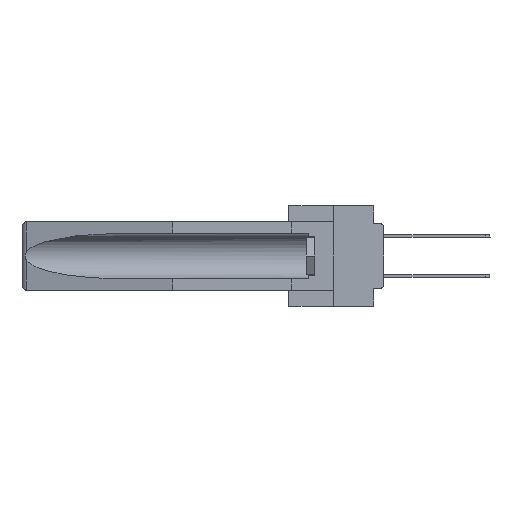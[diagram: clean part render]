
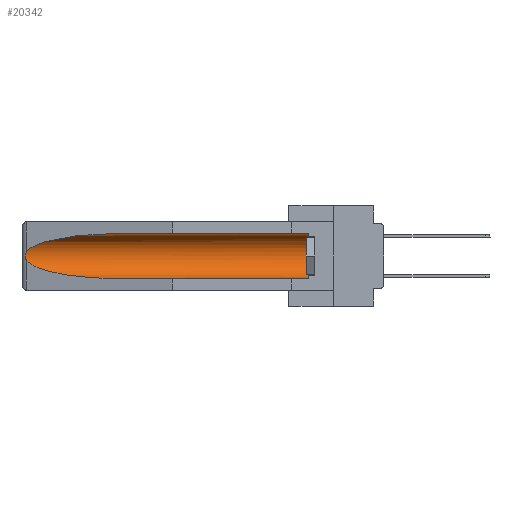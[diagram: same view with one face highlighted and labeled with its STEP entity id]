
A CAD part, left-side view. The second image highlights one B-rep face of the part: STEP entity #20342.
In plain terms, the highlighted cylindrical face has radius 2.857 mm (diameter 5.715 mm), a partial arc.
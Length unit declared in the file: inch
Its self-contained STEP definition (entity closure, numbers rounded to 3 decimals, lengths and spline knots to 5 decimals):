
#303 = CARTESIAN_POINT ( 'NONE',  ( 0.155, 1.07973, -0.284 ) ) ;
#502 = CARTESIAN_POINT ( 'NONE',  ( 0.26655, 1.53094, -0.18657 ) ) ;
#1109 = EDGE_CURVE ( 'NONE', #25879, #15699, #24027, .T. ) ;
#1837 = EDGE_CURVE ( 'NONE', #23606, #25879, #31931, .T. ) ;
#3815 = CARTESIAN_POINT ( 'NONE',  ( 0.2675, 1.53308, -0.17534 ) ) ;
#3900 = CARTESIAN_POINT ( 'NONE',  ( 0.21114, 1.30732, -0.059 ) ) ;
#5561 = CARTESIAN_POINT ( 'NONE',  ( 0.26537, 1.52718, -0.14972 ) ) ;
#5753 = EDGE_CURVE ( 'NONE', #7102, #23606, #14064, .T. ) ;
#6624 = ORIENTED_EDGE ( 'NONE', *, *, #1109, .T. ) ;
#6675 = CARTESIAN_POINT ( 'NONE',  ( 0.155, 1.07973, -0.059 ) ) ;
#7102 = VERTEX_POINT ( 'NONE', #24987 ) ;
#7308 = ORIENTED_EDGE ( 'NONE', *, *, #5753, .T. ) ;
#7435 = LINE ( 'NONE', #27918, #16071 ) ;
#8150 = CYLINDRICAL_SURFACE ( 'NONE', #29173, 0.1125 ) ;
#8556 = FACE_OUTER_BOUND ( 'NONE', #35302, .T. ) ;
#8893 = EDGE_CURVE ( 'NONE', #16748, #29766, #20570, .T. ) ;
#9699 = CARTESIAN_POINT ( 'NONE',  ( 0.26537, 1.52718, -0.14972 ) ) ;
#9883 = EDGE_CURVE ( 'NONE', #29766, #7102, #7435, .T. ) ;
#10340 = CARTESIAN_POINT ( 'NONE',  ( 0.155, 0.126, -0.284 ) ) ;
#11293 = LINE ( 'NONE', #13041, #28548 ) ;
#11971 = CARTESIAN_POINT ( 'NONE',  ( 0.155, 1.07973, -0.284 ) ) ;
#13041 = CARTESIAN_POINT ( 'NONE',  ( 0.155, -0.30754, -0.284 ) ) ;
#13112 = CARTESIAN_POINT ( 'NONE',  ( 0.26537, 1.52718, -0.19328 ) ) ;
#13301 = AXIS2_PLACEMENT_3D ( 'NONE', #13698, #24849, #33728 ) ;
#13698 = CARTESIAN_POINT ( 'NONE',  ( 0.155, 0.126, -0.1715 ) ) ;
#14064 =( BOUNDED_CURVE ( )  B_SPLINE_CURVE ( 3, ( #6675, #3900, #15002, #9699 ),
 .UNSPECIFIED., .F., .T. ) 
 B_SPLINE_CURVE_WITH_KNOTS ( ( 4, 4 ),
 ( 4.71239, 6.08839 ),
 .UNSPECIFIED. ) 
 CURVE ( )  GEOMETRIC_REPRESENTATION_ITEM ( )  RATIONAL_B_SPLINE_CURVE ( ( 1., 0.848, 0.848, 1. ) ) 
 REPRESENTATION_ITEM ( '' )  );
#15002 = CARTESIAN_POINT ( 'NONE',  ( 0.25451, 1.48313, -0.09465 ) ) ;
#15402 = ORIENTED_EDGE ( 'NONE', *, *, #20407, .F. ) ;
#15435 = CARTESIAN_POINT ( 'NONE',  ( 0.26597, 1.5296, -0.19026 ) ) ;
#15699 = VERTEX_POINT ( 'NONE', #11971 ) ;
#15819 = DIRECTION ( 'NONE',  ( 0., 1., 0. ) ) ;
#15994 = DIRECTION ( 'NONE',  ( 0., 1., 0. ) ) ;
#16071 = VECTOR ( 'NONE', #15994, 39.37008 ) ;
#16748 = VERTEX_POINT ( 'NONE', #10340 ) ;
#17665 = CARTESIAN_POINT ( 'NONE',  ( 0.21114, 1.30732, -0.284 ) ) ;
#18365 = CARTESIAN_POINT ( 'NONE',  ( 0.2673, 1.53269, -0.17917 ) ) ;
#20342 = ADVANCED_FACE ( 'NONE', ( #8556 ), #8150, .F. ) ;
#20407 = EDGE_CURVE ( 'NONE', #16748, #15699, #11293, .T. ) ;
#20570 = CIRCLE ( 'NONE', #13301, 0.1125 ) ;
#21153 = CARTESIAN_POINT ( 'NONE',  ( 0.26537, 1.52718, -0.14972 ) ) ;
#21275 = CARTESIAN_POINT ( 'NONE',  ( 0.26597, 1.52961, -0.15275 ) ) ;
#23119 = DIRECTION ( 'NONE',  ( 0., 1., 0. ) ) ;
#23282 = ORIENTED_EDGE ( 'NONE', *, *, #8893, .T. ) ;
#23606 = VERTEX_POINT ( 'NONE', #5561 ) ;
#24027 =( BOUNDED_CURVE ( )  B_SPLINE_CURVE ( 3, ( #35235, #35113, #17665, #303 ),
 .UNSPECIFIED., .F., .F. ) 
 B_SPLINE_CURVE_WITH_KNOTS ( ( 4, 4 ),
 ( 0.1948, 1.5708 ),
 .UNSPECIFIED. ) 
 CURVE ( )  GEOMETRIC_REPRESENTATION_ITEM ( )  RATIONAL_B_SPLINE_CURVE ( ( 1., 0.848, 0.848, 1. ) ) 
 REPRESENTATION_ITEM ( '' )  );
#24849 = DIRECTION ( 'NONE',  ( 0., -1., 0. ) ) ;
#24987 = CARTESIAN_POINT ( 'NONE',  ( 0.155, 1.07973, -0.059 ) ) ;
#25879 = VERTEX_POINT ( 'NONE', #13112 ) ;
#26140 = ORIENTED_EDGE ( 'NONE', *, *, #9883, .T. ) ;
#27918 = CARTESIAN_POINT ( 'NONE',  ( 0.155, -0.30754, -0.059 ) ) ;
#28548 = VECTOR ( 'NONE', #15819, 39.37008 ) ;
#29173 = AXIS2_PLACEMENT_3D ( 'NONE', #34042, #23119, #34394 ) ;
#29766 = VERTEX_POINT ( 'NONE', #34232 ) ;
#31931 = B_SPLINE_CURVE_WITH_KNOTS ( 'NONE', 3,
 ( #21153, #21275, #32796, #35438, #32662, #3815, #18365, #502, #15435, #32529 ),
 .UNSPECIFIED., .F., .F.,
 ( 4, 2, 2, 2, 4 ),
 ( 0., 0.00029, 0.00058, 0.00087, 0.00117 ),
 .UNSPECIFIED. ) ;
#32529 = CARTESIAN_POINT ( 'NONE',  ( 0.26537, 1.52718, -0.19328 ) ) ;
#32662 = CARTESIAN_POINT ( 'NONE',  ( 0.2675, 1.53308, -0.16763 ) ) ;
#32796 = CARTESIAN_POINT ( 'NONE',  ( 0.26654, 1.53092, -0.15636 ) ) ;
#33728 = DIRECTION ( 'NONE',  ( 0., 0., 1. ) ) ;
#34042 = CARTESIAN_POINT ( 'NONE',  ( 0.155, -0.30754, -0.1715 ) ) ;
#34232 = CARTESIAN_POINT ( 'NONE',  ( 0.155, 0.126, -0.059 ) ) ;
#34394 = DIRECTION ( 'NONE',  ( 0., 0., 1. ) ) ;
#35113 = CARTESIAN_POINT ( 'NONE',  ( 0.25451, 1.48313, -0.24835 ) ) ;
#35235 = CARTESIAN_POINT ( 'NONE',  ( 0.26537, 1.52718, -0.19328 ) ) ;
#35302 = EDGE_LOOP ( 'NONE', ( #7308, #35584, #6624, #15402, #23282, #26140 ) ) ;
#35438 = CARTESIAN_POINT ( 'NONE',  ( 0.2673, 1.5327, -0.16383 ) ) ;
#35584 = ORIENTED_EDGE ( 'NONE', *, *, #1837, .T. ) ;
